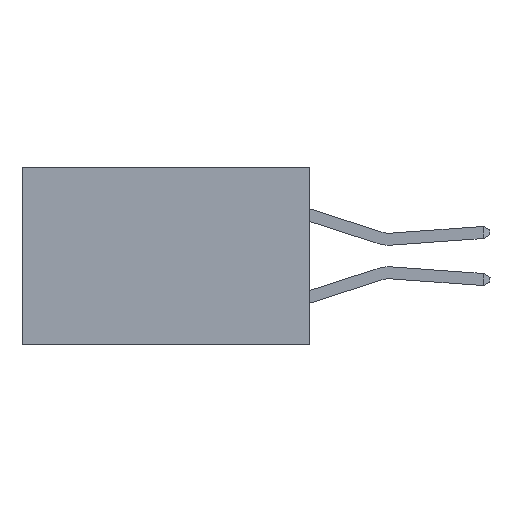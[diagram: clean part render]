
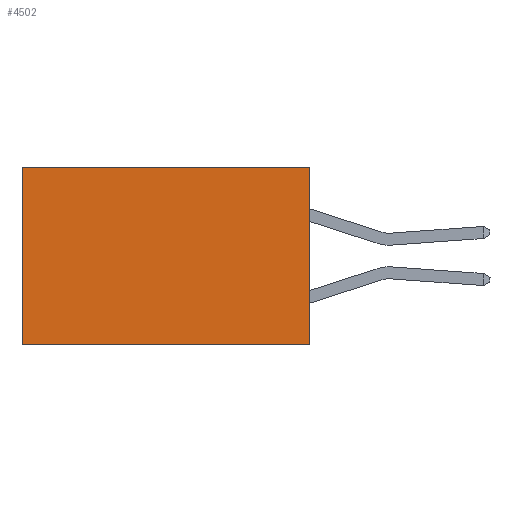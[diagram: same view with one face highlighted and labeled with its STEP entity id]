
A CAD part, left-side view. The second image highlights one B-rep face of the part: STEP entity #4502.
In plain terms, the highlighted planar face has unit normal (-1, 0, 0).
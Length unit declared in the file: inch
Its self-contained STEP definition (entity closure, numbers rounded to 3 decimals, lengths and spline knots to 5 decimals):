
#1226 = PLANE ( 'NONE',  #1815 ) ;
#1815 = AXIS2_PLACEMENT_3D ( 'NONE', #4155, #21428, #20447 ) ;
#2887 = DIRECTION ( 'NONE',  ( 0., 1., 0. ) ) ;
#2972 = CARTESIAN_POINT ( 'NONE',  ( 0.2615, 0.6, -0.37 ) ) ;
#3181 = VERTEX_POINT ( 'NONE', #3819 ) ;
#3819 = CARTESIAN_POINT ( 'NONE',  ( 0.2615, 0., -0.37 ) ) ;
#4018 = EDGE_CURVE ( 'NONE', #15760, #16952, #7932, .T. ) ;
#4155 = CARTESIAN_POINT ( 'NONE',  ( 0.2615, 0., -0.37 ) ) ;
#4502 = ADVANCED_FACE ( 'NONE', ( #6782 ), #1226, .F. ) ;
#5979 = CARTESIAN_POINT ( 'NONE',  ( 0.2615, 0., -0.37 ) ) ;
#6642 = VECTOR ( 'NONE', #9310, 39.37008 ) ;
#6782 = FACE_OUTER_BOUND ( 'NONE', #9789, .T. ) ;
#7932 = LINE ( 'NONE', #2972, #17439 ) ;
#8053 = ORIENTED_EDGE ( 'NONE', *, *, #8512, .F. ) ;
#8333 = LINE ( 'NONE', #5979, #13099 ) ;
#8505 = ORIENTED_EDGE ( 'NONE', *, *, #17004, .T. ) ;
#8512 = EDGE_CURVE ( 'NONE', #9644, #3181, #8333, .T. ) ;
#9310 = DIRECTION ( 'NONE',  ( 0., 1., 0. ) ) ;
#9644 = VERTEX_POINT ( 'NONE', #12823 ) ;
#9789 = EDGE_LOOP ( 'NONE', ( #16229, #10046, #8053, #8505 ) ) ;
#10046 = ORIENTED_EDGE ( 'NONE', *, *, #20031, .F. ) ;
#11206 = DIRECTION ( 'NONE',  ( 0., 0., -1. ) ) ;
#12098 = CARTESIAN_POINT ( 'NONE',  ( 0.2615, 0.6, 0. ) ) ;
#12823 = CARTESIAN_POINT ( 'NONE',  ( 0.2615, 0., 0. ) ) ;
#13099 = VECTOR ( 'NONE', #14913, 39.37008 ) ;
#14711 = CARTESIAN_POINT ( 'NONE',  ( 0.2615, 0., -0.37 ) ) ;
#14913 = DIRECTION ( 'NONE',  ( 0., 0., -1. ) ) ;
#15010 = LINE ( 'NONE', #17260, #15572 ) ;
#15572 = VECTOR ( 'NONE', #2887, 39.37008 ) ;
#15760 = VERTEX_POINT ( 'NONE', #12098 ) ;
#16229 = ORIENTED_EDGE ( 'NONE', *, *, #4018, .T. ) ;
#16952 = VERTEX_POINT ( 'NONE', #17186 ) ;
#17004 = EDGE_CURVE ( 'NONE', #9644, #15760, #15010, .T. ) ;
#17186 = CARTESIAN_POINT ( 'NONE',  ( 0.2615, 0.6, -0.37 ) ) ;
#17260 = CARTESIAN_POINT ( 'NONE',  ( 0.2615, 0., 0. ) ) ;
#17439 = VECTOR ( 'NONE', #11206, 39.37008 ) ;
#20031 = EDGE_CURVE ( 'NONE', #3181, #16952, #20866, .T. ) ;
#20447 = DIRECTION ( 'NONE',  ( 0., 0., -1. ) ) ;
#20866 = LINE ( 'NONE', #14711, #6642 ) ;
#21428 = DIRECTION ( 'NONE',  ( 1., 0., 0. ) ) ;
